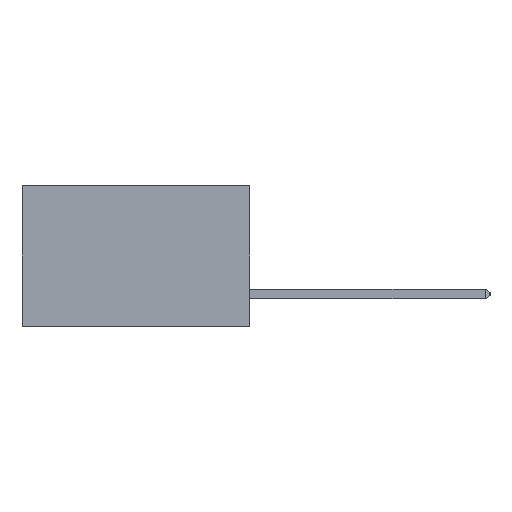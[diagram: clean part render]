
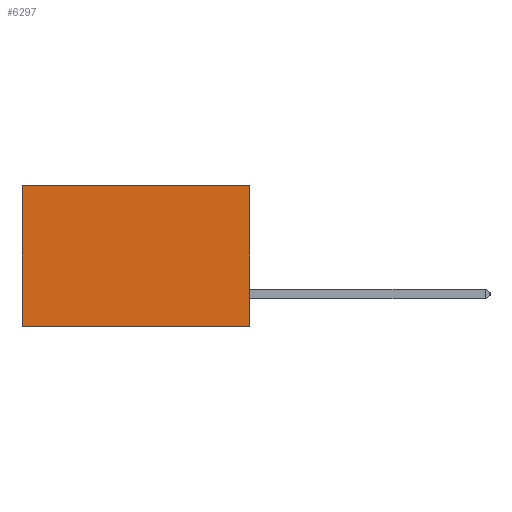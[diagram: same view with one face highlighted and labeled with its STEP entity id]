
A CAD part, left-side view. The second image highlights one B-rep face of the part: STEP entity #6297.
In plain terms, the highlighted planar face has unit normal (-1, 0, 0).
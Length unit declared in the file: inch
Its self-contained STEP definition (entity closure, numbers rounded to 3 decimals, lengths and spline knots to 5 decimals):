
#1067 = CARTESIAN_POINT ( 'NONE',  ( 0.2875, 0., 0. ) ) ;
#1823 = CARTESIAN_POINT ( 'NONE',  ( 0.2875, 0.6, 0. ) ) ;
#5663 = DIRECTION ( 'NONE',  ( 0., 1., 0. ) ) ;
#6297 = ADVANCED_FACE ( 'NONE', ( #38081 ), #32210, .F. ) ;
#7734 = VECTOR ( 'NONE', #31267, 39.37008 ) ;
#8300 = ORIENTED_EDGE ( 'NONE', *, *, #30284, .T. ) ;
#9209 = CARTESIAN_POINT ( 'NONE',  ( 0.2875, 0., 0. ) ) ;
#9997 = VECTOR ( 'NONE', #20011, 39.37008 ) ;
#12330 = CARTESIAN_POINT ( 'NONE',  ( 0.2875, 0., -0.37 ) ) ;
#12629 = VECTOR ( 'NONE', #25130, 39.37008 ) ;
#12660 = ORIENTED_EDGE ( 'NONE', *, *, #15765, .F. ) ;
#13550 = VECTOR ( 'NONE', #5663, 39.37008 ) ;
#14406 = CARTESIAN_POINT ( 'NONE',  ( 0.2875, 0., 0. ) ) ;
#14744 = EDGE_CURVE ( 'NONE', #33131, #38186, #36269, .T. ) ;
#15303 = VERTEX_POINT ( 'NONE', #24566 ) ;
#15622 = VERTEX_POINT ( 'NONE', #1823 ) ;
#15765 = EDGE_CURVE ( 'NONE', #38186, #15303, #29358, .T. ) ;
#17001 = CARTESIAN_POINT ( 'NONE',  ( 0.2875, 0., 0. ) ) ;
#17405 = DIRECTION ( 'NONE',  ( 1., 0., 0. ) ) ;
#19341 = ORIENTED_EDGE ( 'NONE', *, *, #28870, .T. ) ;
#20011 = DIRECTION ( 'NONE',  ( 0., 1., 0. ) ) ;
#22257 = AXIS2_PLACEMENT_3D ( 'NONE', #14406, #17405, #38090 ) ;
#23633 = CARTESIAN_POINT ( 'NONE',  ( 0.2875, 0., -0.37 ) ) ;
#23667 = LINE ( 'NONE', #28290, #7734 ) ;
#24008 = ORIENTED_EDGE ( 'NONE', *, *, #14744, .F. ) ;
#24566 = CARTESIAN_POINT ( 'NONE',  ( 0.2875, 0.6, -0.37 ) ) ;
#25130 = DIRECTION ( 'NONE',  ( 0., 0., -1. ) ) ;
#27082 = EDGE_LOOP ( 'NONE', ( #19341, #12660, #24008, #8300 ) ) ;
#28290 = CARTESIAN_POINT ( 'NONE',  ( 0.2875, 0.6, 0. ) ) ;
#28870 = EDGE_CURVE ( 'NONE', #15622, #15303, #23667, .T. ) ;
#29358 = LINE ( 'NONE', #23633, #13550 ) ;
#30284 = EDGE_CURVE ( 'NONE', #33131, #15622, #32831, .T. ) ;
#31267 = DIRECTION ( 'NONE',  ( 0., 0., -1. ) ) ;
#32210 = PLANE ( 'NONE',  #22257 ) ;
#32831 = LINE ( 'NONE', #17001, #9997 ) ;
#33131 = VERTEX_POINT ( 'NONE', #9209 ) ;
#36269 = LINE ( 'NONE', #1067, #12629 ) ;
#38081 = FACE_OUTER_BOUND ( 'NONE', #27082, .T. ) ;
#38090 = DIRECTION ( 'NONE',  ( 0., 0., -1. ) ) ;
#38186 = VERTEX_POINT ( 'NONE', #12330 ) ;
